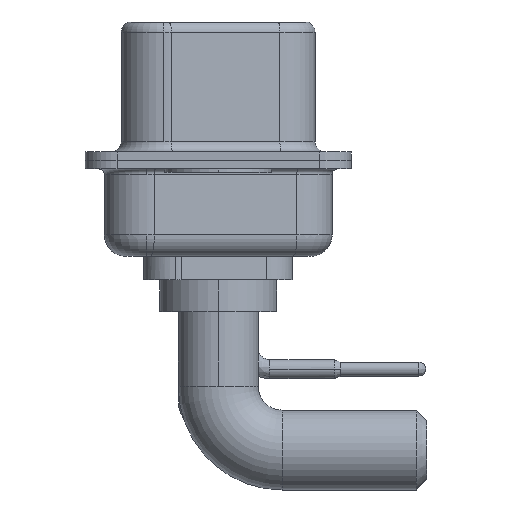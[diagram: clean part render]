
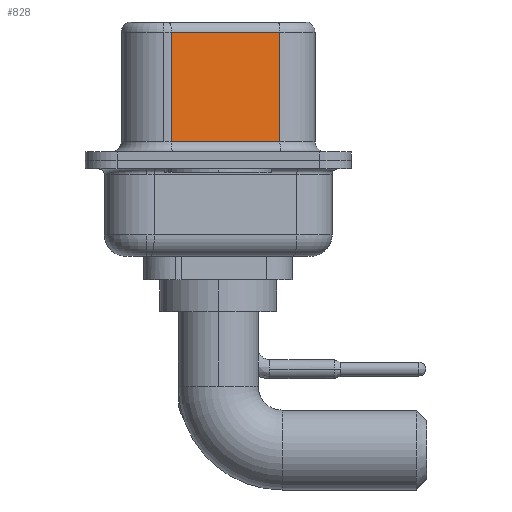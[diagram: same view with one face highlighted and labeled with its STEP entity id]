
A CAD part, left-side view. The second image highlights one B-rep face of the part: STEP entity #828.
In plain terms, the highlighted planar face has unit normal (-0.985, -0.174, 0).
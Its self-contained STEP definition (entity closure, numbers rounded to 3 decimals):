
#187 = VECTOR ( 'NONE', #17762, 1000. ) ;
#766 = ORIENTED_EDGE ( 'NONE', *, *, #21414, .F. ) ;
#828 = ADVANCED_FACE ( 'NONE', ( #6478 ), #8127, .F. ) ;
#999 = ORIENTED_EDGE ( 'NONE', *, *, #9733, .T. ) ;
#1214 = CARTESIAN_POINT ( 'NONE',  ( 4.58, -2.897, 6.02 ) ) ;
#1363 = EDGE_CURVE ( 'NONE', #6380, #16141, #7987, .T. ) ;
#1585 = DIRECTION ( 'NONE',  ( 0., 0., -1. ) ) ;
#1821 = CARTESIAN_POINT ( 'NONE',  ( 4.58, -2.897, 6.02 ) ) ;
#3156 = DIRECTION ( 'NONE',  ( -0.174, 0.985, 0. ) ) ;
#3626 = VECTOR ( 'NONE', #4744, 1000. ) ;
#4425 = LINE ( 'NONE', #16011, #187 ) ;
#4676 = CARTESIAN_POINT ( 'NONE',  ( 3.68, 2.203, 6.52 ) ) ;
#4744 = DIRECTION ( 'NONE',  ( -0.174, 0.985, 0. ) ) ;
#4748 = EDGE_LOOP ( 'NONE', ( #766, #18989, #6808, #999 ) ) ;
#4885 = AXIS2_PLACEMENT_3D ( 'NONE', #14859, #21675, #3156 ) ;
#6380 = VERTEX_POINT ( 'NONE', #21613 ) ;
#6478 = FACE_OUTER_BOUND ( 'NONE', #4748, .T. ) ;
#6622 = LINE ( 'NONE', #1214, #3626 ) ;
#6808 = ORIENTED_EDGE ( 'NONE', *, *, #1363, .T. ) ;
#6899 = CARTESIAN_POINT ( 'NONE',  ( 3.68, 2.203, 0.9 ) ) ;
#7987 = LINE ( 'NONE', #4676, #8436 ) ;
#8127 = PLANE ( 'NONE',  #4885 ) ;
#8436 = VECTOR ( 'NONE', #1585, 1000. ) ;
#9733 = EDGE_CURVE ( 'NONE', #16141, #16182, #4425, .T. ) ;
#13255 = DIRECTION ( 'NONE',  ( 0., 0., -1. ) ) ;
#14075 = CARTESIAN_POINT ( 'NONE',  ( 4.58, -2.897, 0.9 ) ) ;
#14859 = CARTESIAN_POINT ( 'NONE',  ( 4.58, -2.897, 6.52 ) ) ;
#16011 = CARTESIAN_POINT ( 'NONE',  ( 4.58, -2.897, 0.9 ) ) ;
#16141 = VERTEX_POINT ( 'NONE', #6899 ) ;
#16182 = VERTEX_POINT ( 'NONE', #14075 ) ;
#16655 = VECTOR ( 'NONE', #13255, 1000. ) ;
#17762 = DIRECTION ( 'NONE',  ( 0.174, -0.985, 0. ) ) ;
#17962 = CARTESIAN_POINT ( 'NONE',  ( 4.58, -2.897, 6.52 ) ) ;
#18300 = LINE ( 'NONE', #17962, #16655 ) ;
#18989 = ORIENTED_EDGE ( 'NONE', *, *, #19576, .T. ) ;
#19154 = VERTEX_POINT ( 'NONE', #1821 ) ;
#19576 = EDGE_CURVE ( 'NONE', #19154, #6380, #6622, .T. ) ;
#21414 = EDGE_CURVE ( 'NONE', #19154, #16182, #18300, .T. ) ;
#21613 = CARTESIAN_POINT ( 'NONE',  ( 3.68, 2.203, 6.02 ) ) ;
#21675 = DIRECTION ( 'NONE',  ( 0.985, 0.174, 0. ) ) ;
